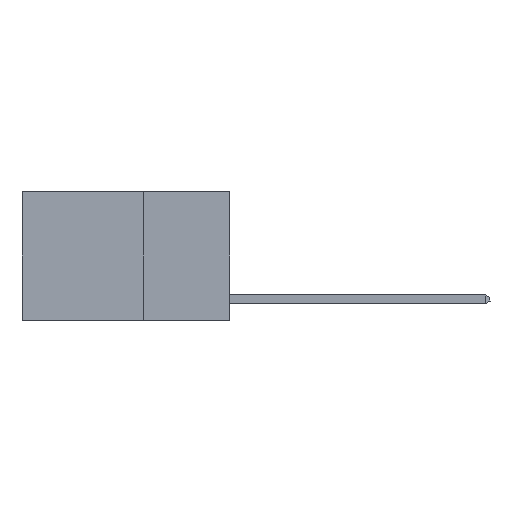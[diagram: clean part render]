
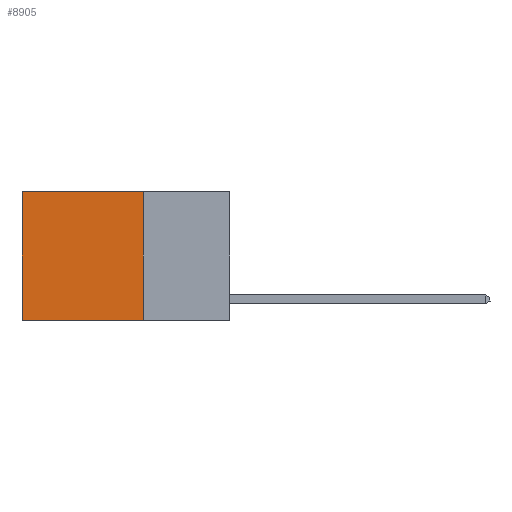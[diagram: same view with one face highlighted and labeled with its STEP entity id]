
A CAD part, left-side view. The second image highlights one B-rep face of the part: STEP entity #8905.
In plain terms, the highlighted planar face has unit normal (-1, 0, 0).
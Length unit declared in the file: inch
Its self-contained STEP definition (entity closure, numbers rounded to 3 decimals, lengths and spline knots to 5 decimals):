
#258 = VERTEX_POINT ( 'NONE', #700 ) ;
#536 = VERTEX_POINT ( 'NONE', #16504 ) ;
#700 = CARTESIAN_POINT ( 'NONE',  ( 0.2625, 0.6, 0. ) ) ;
#938 = LINE ( 'NONE', #13331, #11879 ) ;
#1157 = CARTESIAN_POINT ( 'NONE',  ( 0.2625, 0.25, -0.37 ) ) ;
#1202 = EDGE_CURVE ( 'NONE', #3450, #536, #10785, .T. ) ;
#2984 = ORIENTED_EDGE ( 'NONE', *, *, #6881, .T. ) ;
#2999 = DIRECTION ( 'NONE',  ( 1., 0., 0. ) ) ;
#3357 = ORIENTED_EDGE ( 'NONE', *, *, #1202, .F. ) ;
#3450 = VERTEX_POINT ( 'NONE', #1157 ) ;
#3545 = VERTEX_POINT ( 'NONE', #5372 ) ;
#4186 = PLANE ( 'NONE',  #4467 ) ;
#4467 = AXIS2_PLACEMENT_3D ( 'NONE', #15417, #2999, #8594 ) ;
#5059 = EDGE_CURVE ( 'NONE', #3545, #258, #13742, .T. ) ;
#5372 = CARTESIAN_POINT ( 'NONE',  ( 0.2625, 0.25, 0. ) ) ;
#5821 = DIRECTION ( 'NONE',  ( 0., 1., 0. ) ) ;
#6424 = ORIENTED_EDGE ( 'NONE', *, *, #8679, .F. ) ;
#6505 = DIRECTION ( 'NONE',  ( 0., 0., -1. ) ) ;
#6881 = EDGE_CURVE ( 'NONE', #258, #536, #938, .T. ) ;
#8143 = DIRECTION ( 'NONE',  ( 0., 0., -1. ) ) ;
#8182 = CARTESIAN_POINT ( 'NONE',  ( 0.2625, 0.25, -0.37 ) ) ;
#8290 = EDGE_LOOP ( 'NONE', ( #2984, #3357, #6424, #16343 ) ) ;
#8594 = DIRECTION ( 'NONE',  ( 0., 0., -1. ) ) ;
#8679 = EDGE_CURVE ( 'NONE', #3545, #3450, #9415, .T. ) ;
#8905 = ADVANCED_FACE ( 'NONE', ( #15323 ), #4186, .F. ) ;
#9415 = LINE ( 'NONE', #17669, #10777 ) ;
#10777 = VECTOR ( 'NONE', #8143, 39.37008 ) ;
#10785 = LINE ( 'NONE', #8182, #12957 ) ;
#11879 = VECTOR ( 'NONE', #6505, 39.37008 ) ;
#12385 = CARTESIAN_POINT ( 'NONE',  ( 0.2625, 0.25, 0. ) ) ;
#12957 = VECTOR ( 'NONE', #16438, 39.37008 ) ;
#13331 = CARTESIAN_POINT ( 'NONE',  ( 0.2625, 0.6, 0. ) ) ;
#13742 = LINE ( 'NONE', #12385, #14387 ) ;
#14387 = VECTOR ( 'NONE', #5821, 39.37008 ) ;
#15323 = FACE_OUTER_BOUND ( 'NONE', #8290, .T. ) ;
#15417 = CARTESIAN_POINT ( 'NONE',  ( 0.2625, 0.25, 0. ) ) ;
#16343 = ORIENTED_EDGE ( 'NONE', *, *, #5059, .T. ) ;
#16438 = DIRECTION ( 'NONE',  ( 0., 1., 0. ) ) ;
#16504 = CARTESIAN_POINT ( 'NONE',  ( 0.2625, 0.6, -0.37 ) ) ;
#17669 = CARTESIAN_POINT ( 'NONE',  ( 0.2625, 0.25, 0. ) ) ;
